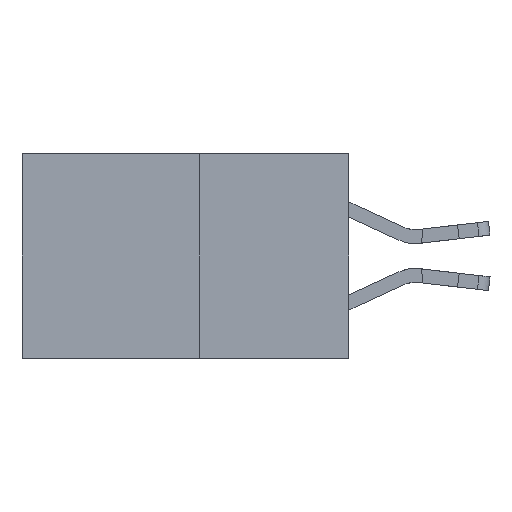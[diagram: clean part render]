
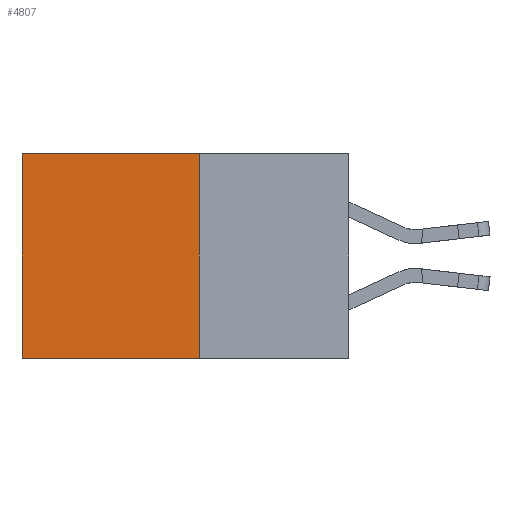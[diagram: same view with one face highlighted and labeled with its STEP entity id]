
A CAD part, left-side view. The second image highlights one B-rep face of the part: STEP entity #4807.
In plain terms, the highlighted planar face has unit normal (-1, 0, 0).
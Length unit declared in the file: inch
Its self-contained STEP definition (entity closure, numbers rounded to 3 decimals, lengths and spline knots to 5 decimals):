
#497 = DIRECTION ( 'NONE',  ( 0., 1., 0. ) ) ;
#520 = LINE ( 'NONE', #3604, #11315 ) ;
#680 = DIRECTION ( 'NONE',  ( 0., 1., 0. ) ) ;
#918 = CARTESIAN_POINT ( 'NONE',  ( 0.277, 0.27, -0.37 ) ) ;
#1411 = VERTEX_POINT ( 'NONE', #3715 ) ;
#1562 = EDGE_CURVE ( 'NONE', #1411, #2260, #10490, .T. ) ;
#1688 = ORIENTED_EDGE ( 'NONE', *, *, #1562, .T. ) ;
#2260 = VERTEX_POINT ( 'NONE', #3555 ) ;
#2512 = EDGE_CURVE ( 'NONE', #2260, #5506, #4839, .T. ) ;
#2582 = AXIS2_PLACEMENT_3D ( 'NONE', #7693, #7060, #7029 ) ;
#2876 = FACE_OUTER_BOUND ( 'NONE', #7157, .T. ) ;
#3326 = DIRECTION ( 'NONE',  ( 0., 0., -1. ) ) ;
#3390 = LINE ( 'NONE', #918, #9010 ) ;
#3555 = CARTESIAN_POINT ( 'NONE',  ( 0.277, 0.59, 0. ) ) ;
#3604 = CARTESIAN_POINT ( 'NONE',  ( 0.277, 0.27, -0.37 ) ) ;
#3715 = CARTESIAN_POINT ( 'NONE',  ( 0.277, 0.27, 0. ) ) ;
#4097 = ORIENTED_EDGE ( 'NONE', *, *, #4567, .F. ) ;
#4151 = VECTOR ( 'NONE', #7763, 39.37008 ) ;
#4384 = CARTESIAN_POINT ( 'NONE',  ( 0.277, 0.27, 0. ) ) ;
#4567 = EDGE_CURVE ( 'NONE', #9110, #5506, #3390, .T. ) ;
#4807 = ADVANCED_FACE ( 'NONE', ( #2876 ), #7180, .F. ) ;
#4839 = LINE ( 'NONE', #5132, #4151 ) ;
#5132 = CARTESIAN_POINT ( 'NONE',  ( 0.277, 0.59, -0.37 ) ) ;
#5353 = VECTOR ( 'NONE', #497, 39.37008 ) ;
#5506 = VERTEX_POINT ( 'NONE', #8894 ) ;
#7029 = DIRECTION ( 'NONE',  ( 0., 0., -1. ) ) ;
#7060 = DIRECTION ( 'NONE',  ( 1., 0., 0. ) ) ;
#7157 = EDGE_LOOP ( 'NONE', ( #10560, #4097, #10258, #1688 ) ) ;
#7180 = PLANE ( 'NONE',  #2582 ) ;
#7693 = CARTESIAN_POINT ( 'NONE',  ( 0.277, 0.27, -0.37 ) ) ;
#7763 = DIRECTION ( 'NONE',  ( 0., 0., -1. ) ) ;
#8367 = CARTESIAN_POINT ( 'NONE',  ( 0.277, 0.27, -0.37 ) ) ;
#8894 = CARTESIAN_POINT ( 'NONE',  ( 0.277, 0.59, -0.37 ) ) ;
#9010 = VECTOR ( 'NONE', #680, 39.37008 ) ;
#9110 = VERTEX_POINT ( 'NONE', #8367 ) ;
#10192 = EDGE_CURVE ( 'NONE', #1411, #9110, #520, .T. ) ;
#10258 = ORIENTED_EDGE ( 'NONE', *, *, #10192, .F. ) ;
#10490 = LINE ( 'NONE', #4384, #5353 ) ;
#10560 = ORIENTED_EDGE ( 'NONE', *, *, #2512, .T. ) ;
#11315 = VECTOR ( 'NONE', #3326, 39.37008 ) ;
